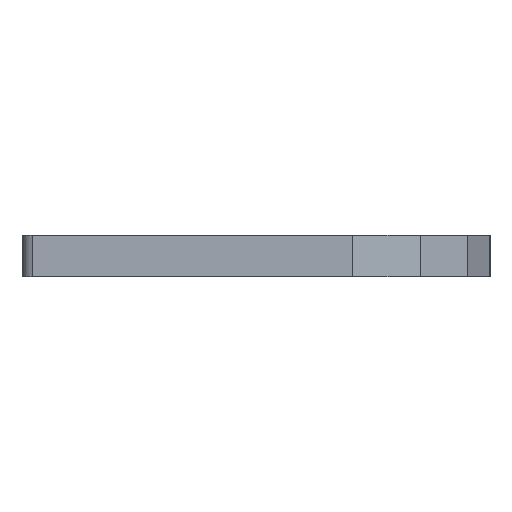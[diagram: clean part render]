
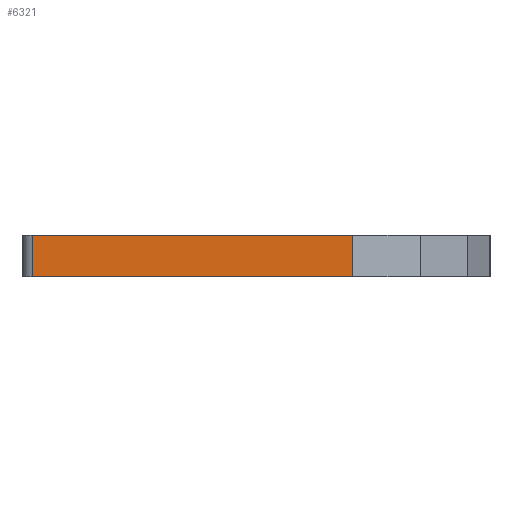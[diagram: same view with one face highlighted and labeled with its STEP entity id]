
A CAD part, left-side view. The second image highlights one B-rep face of the part: STEP entity #6321.
In plain terms, the highlighted planar face has unit normal (-1, 0, 0).
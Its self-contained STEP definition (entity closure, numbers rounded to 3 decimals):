
#684 = EDGE_CURVE ( 'NONE', #9027, #10220, #6637, .T. ) ;
#685 = EDGE_CURVE ( 'NONE', #6700, #9027, #6216, .T. ) ;
#688 = EDGE_CURVE ( 'NONE', #6406, #10220, #6228, .T. ) ;
#697 = EDGE_CURVE ( 'NONE', #6700, #6406, #6352, .T. ) ;
#1491 = ORIENTED_EDGE ( 'NONE', *, *, #688, .F. ) ;
#3378 = CARTESIAN_POINT ( 'NONE',  ( -62.408, -19.739, 0. ) ) ;
#3822 = DIRECTION ( 'NONE',  ( 0., 0., -1. ) ) ;
#3867 = CARTESIAN_POINT ( 'NONE',  ( -62.408, -19.739, 0.203 ) ) ;
#3909 = DIRECTION ( 'NONE',  ( 0., 0., -1. ) ) ;
#3920 = DIRECTION ( 'NONE',  ( 0., -1., 0. ) ) ;
#3940 = CARTESIAN_POINT ( 'NONE',  ( -62.408, -21.323, 0.203 ) ) ;
#3953 = CARTESIAN_POINT ( 'NONE',  ( -62.408, -19.739, 0.203 ) ) ;
#3976 = DIRECTION ( 'NONE',  ( 0., -1., 0. ) ) ;
#4542 = CARTESIAN_POINT ( 'NONE',  ( -62.408, -19.739, 0. ) ) ;
#5861 = CARTESIAN_POINT ( 'NONE',  ( -62.408, -19.739, 0.203 ) ) ;
#6045 = VECTOR ( 'NONE', #3920, 1000. ) ;
#6070 = VECTOR ( 'NONE', #3822, 1000. ) ;
#6203 = VECTOR ( 'NONE', #3909, 1000. ) ;
#6216 = LINE ( 'NONE', #3953, #6203 ) ;
#6228 = LINE ( 'NONE', #3940, #6070 ) ;
#6321 = ADVANCED_FACE ( 'NONE', ( #10250 ), #8400, .F. ) ;
#6341 = VECTOR ( 'NONE', #3976, 1000. ) ;
#6352 = LINE ( 'NONE', #3867, #6045 ) ;
#6406 = VERTEX_POINT ( 'NONE', #7739 ) ;
#6637 = LINE ( 'NONE', #4542, #6341 ) ;
#6696 = ORIENTED_EDGE ( 'NONE', *, *, #697, .F. ) ;
#6700 = VERTEX_POINT ( 'NONE', #5861 ) ;
#7739 = CARTESIAN_POINT ( 'NONE',  ( -62.408, -21.323, 0.203 ) ) ;
#8323 = DIRECTION ( 'NONE',  ( 0., 0., -1. ) ) ;
#8334 = DIRECTION ( 'NONE',  ( 1., 0., 0. ) ) ;
#8362 = CARTESIAN_POINT ( 'NONE',  ( -62.408, -19.739, 0.203 ) ) ;
#8400 = PLANE ( 'NONE',  #11377 ) ;
#8908 = CARTESIAN_POINT ( 'NONE',  ( -62.408, -21.323, 0. ) ) ;
#9027 = VERTEX_POINT ( 'NONE', #3378 ) ;
#9327 = ORIENTED_EDGE ( 'NONE', *, *, #685, .T. ) ;
#9643 = EDGE_LOOP ( 'NONE', ( #10806, #1491, #6696, #9327 ) ) ;
#10220 = VERTEX_POINT ( 'NONE', #8908 ) ;
#10250 = FACE_OUTER_BOUND ( 'NONE', #9643, .T. ) ;
#10806 = ORIENTED_EDGE ( 'NONE', *, *, #684, .T. ) ;
#11377 = AXIS2_PLACEMENT_3D ( 'NONE', #8362, #8334, #8323 ) ;
